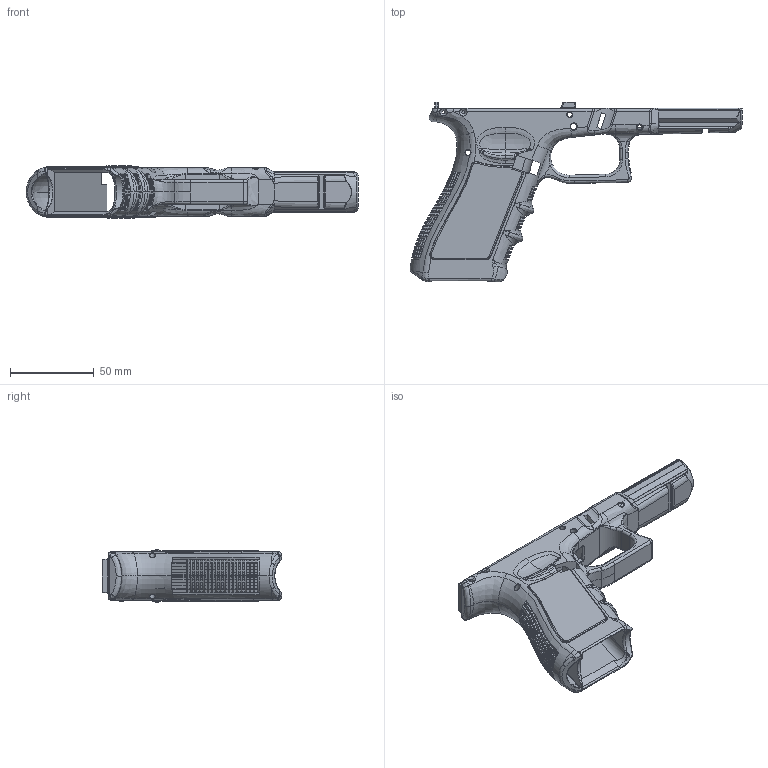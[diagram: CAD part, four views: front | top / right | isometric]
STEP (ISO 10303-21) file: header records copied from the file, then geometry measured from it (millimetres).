
FILE_DESCRIPTION(/* description */ (''),/* implementation_level */ '2;1');
FILE_NAME(/* name */ 'FreeMan''s G17 Frame - countersunk (tapered) screws.stp',/* time_stamp */ '2019-03-17T16:24:20-05:00',/* author */ ('johne'),/* organization */ (''),/* preprocessor_version */ 'ST-DEVELOPER v16.13',/* originating_system */ 'Autodesk Inventor 2018',/* authorisation */ '');
FILE_SCHEMA (('AUTOMOTIVE_DESIGN { 1 0 10303 214 3 1 1 }'));
Products named in the file (1): 3D PRINTED 17-RECEIVER SECOND MODEL Rear Mod Copy v7
Bounding box: 197.79 x 107 x 31.4 mm (x, y, z)
Volume: 82356.1 mm3; surface area: 51699.7 mm2
Topology: 1 solids, 1 shells, 2516 faces, 6928 edges, 4386 vertices
Faces by surface type: bspline 1115, plane 845, cylinder 463, torus 37, cone 33, sphere 23
Full cylindrical faces by diameter (mm): 2 x4, 3 x5, 3.2 x2, 3.8 x2
Entity records: 186434 total; most frequent: CARTESIAN_POINT 128159, ORIENTED_EDGE 13726, DIRECTION 10506, EDGE_CURVE 6863, VERTEX_POINT 4366, AXIS2_PLACEMENT_3D 3889, LINE 2728, VECTOR 2728
